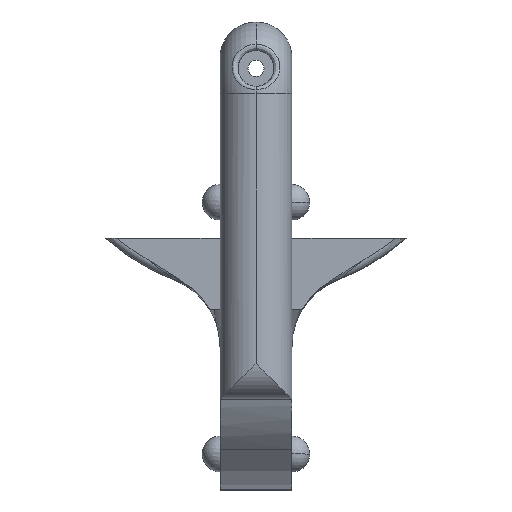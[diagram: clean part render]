
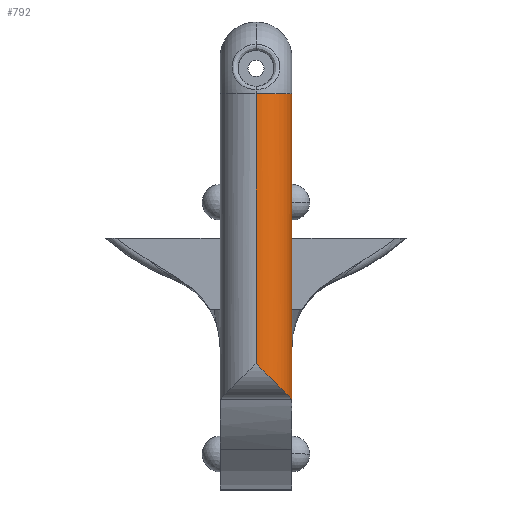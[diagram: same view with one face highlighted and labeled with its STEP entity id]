
A CAD part, top view. The second image highlights one B-rep face of the part: STEP entity #792.
In plain terms, the highlighted cylindrical face has radius 5 mm (diameter 10 mm), a partial arc.
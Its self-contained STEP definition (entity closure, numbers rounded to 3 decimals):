
#147 = CARTESIAN_POINT ( 'NONE',  ( 9.998, -12.563, 67.629 ) ) ;
#154 = CARTESIAN_POINT ( 'NONE',  ( 5., -7.564, 72.5 ) ) ;
#159 = CARTESIAN_POINT ( 'NONE',  ( 10., 30., 67.5 ) ) ;
#161 = DIRECTION ( 'NONE',  ( 0., 0., 1. ) ) ;
#172 = DIRECTION ( 'NONE',  ( 0., -1., 0. ) ) ;
#261 = CARTESIAN_POINT ( 'NONE',  ( 10., -12.565, 67.543 ) ) ;
#276 = VERTEX_POINT ( 'NONE', #154 ) ;
#401 = CARTESIAN_POINT ( 'NONE',  ( 10., -12.566, 67.5 ) ) ;
#425 = EDGE_CURVE ( 'NONE', #1473, #722, #1777, .T. ) ;
#447 =( BOUNDED_CURVE ( )  B_SPLINE_CURVE ( 3, ( #147, #660, #1488, #492 ),
 .UNSPECIFIED., .F., .T. ) 
 B_SPLINE_CURVE_WITH_KNOTS ( ( 4, 4 ),
 ( 3.167, 4.712 ),
 .UNSPECIFIED. ) 
 CURVE ( )  GEOMETRIC_REPRESENTATION_ITEM ( )  RATIONAL_B_SPLINE_CURVE ( ( 1., 0.811, 0.811, 1. ) ) 
 REPRESENTATION_ITEM ( '' )  );
#492 = CARTESIAN_POINT ( 'NONE',  ( 5., -7.564, 72.5 ) ) ;
#497 = CARTESIAN_POINT ( 'NONE',  ( 5., 0., 72.5 ) ) ;
#519 = ORIENTED_EDGE ( 'NONE', *, *, #626, .F. ) ;
#600 = CIRCLE ( 'NONE', #855, 5. ) ;
#626 = EDGE_CURVE ( 'NONE', #722, #276, #447, .T. ) ;
#660 = CARTESIAN_POINT ( 'NONE',  ( 9.924, -12.489, 70.497 ) ) ;
#683 = CARTESIAN_POINT ( 'NONE',  ( 5., 0., 67.5 ) ) ;
#685 = EDGE_CURVE ( 'NONE', #1615, #782, #600, .T. ) ;
#702 = EDGE_CURVE ( 'NONE', #276, #1615, #1466, .T. ) ;
#722 = VERTEX_POINT ( 'NONE', #1979 ) ;
#782 = VERTEX_POINT ( 'NONE', #159 ) ;
#788 = CARTESIAN_POINT ( 'NONE',  ( 9.998, -12.563, 67.629 ) ) ;
#792 = ADVANCED_FACE ( 'NONE', ( #2126 ), #1225, .T. ) ;
#855 = AXIS2_PLACEMENT_3D ( 'NONE', #2146, #1181, #161 ) ;
#861 = DIRECTION ( 'NONE',  ( 0., 0., 1. ) ) ;
#906 = VECTOR ( 'NONE', #172, 1000. ) ;
#913 = ORIENTED_EDGE ( 'NONE', *, *, #685, .F. ) ;
#960 = LINE ( 'NONE', #1345, #906 ) ;
#990 = VECTOR ( 'NONE', #1334, 1000. ) ;
#1181 = DIRECTION ( 'NONE',  ( 0., 1., 0. ) ) ;
#1225 = CYLINDRICAL_SURFACE ( 'NONE', #1739, 5. ) ;
#1244 = CARTESIAN_POINT ( 'NONE',  ( 5., 30., 72.5 ) ) ;
#1258 = ORIENTED_EDGE ( 'NONE', *, *, #425, .F. ) ;
#1334 = DIRECTION ( 'NONE',  ( 0., 1., 0. ) ) ;
#1345 = CARTESIAN_POINT ( 'NONE',  ( 10., 0., 67.5 ) ) ;
#1429 = CARTESIAN_POINT ( 'NONE',  ( 10., -12.566, 67.5 ) ) ;
#1466 = LINE ( 'NONE', #497, #990 ) ;
#1473 = VERTEX_POINT ( 'NONE', #401 ) ;
#1488 = CARTESIAN_POINT ( 'NONE',  ( 7.869, -10.434, 72.5 ) ) ;
#1511 = ORIENTED_EDGE ( 'NONE', *, *, #702, .F. ) ;
#1615 = VERTEX_POINT ( 'NONE', #1244 ) ;
#1648 = EDGE_CURVE ( 'NONE', #782, #1473, #960, .T. ) ;
#1739 = AXIS2_PLACEMENT_3D ( 'NONE', #683, #1999, #861 ) ;
#1766 = CARTESIAN_POINT ( 'NONE',  ( 9.999, -12.564, 67.586 ) ) ;
#1777 = B_SPLINE_CURVE_WITH_KNOTS ( 'NONE', 3,
 ( #1429, #261, #1766, #788 ),
 .UNSPECIFIED., .F., .F.,
 ( 4, 4 ),
 ( 0., 0. ),
 .UNSPECIFIED. ) ;
#1979 = CARTESIAN_POINT ( 'NONE',  ( 9.998, -12.563, 67.629 ) ) ;
#1999 = DIRECTION ( 'NONE',  ( 0., 1., 0. ) ) ;
#2107 = EDGE_LOOP ( 'NONE', ( #519, #1258, #2155, #913, #1511 ) ) ;
#2126 = FACE_OUTER_BOUND ( 'NONE', #2107, .T. ) ;
#2146 = CARTESIAN_POINT ( 'NONE',  ( 5., 30., 67.5 ) ) ;
#2155 = ORIENTED_EDGE ( 'NONE', *, *, #1648, .F. ) ;
